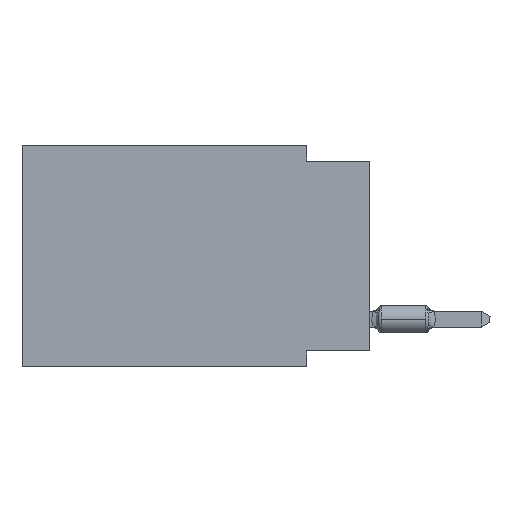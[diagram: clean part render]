
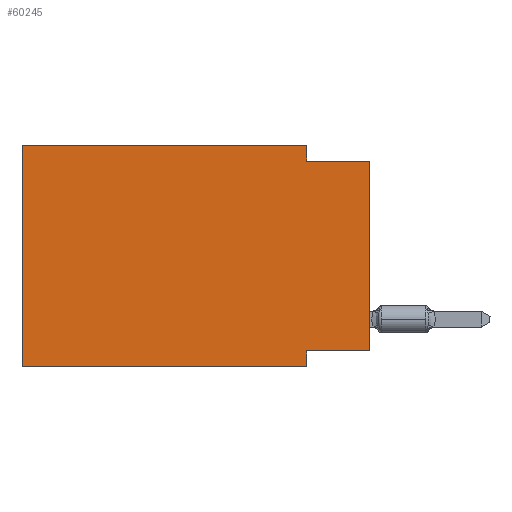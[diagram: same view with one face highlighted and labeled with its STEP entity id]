
A CAD part, left-side view. The second image highlights one B-rep face of the part: STEP entity #60245.
In plain terms, the highlighted planar face has unit normal (-1, 0, 0).
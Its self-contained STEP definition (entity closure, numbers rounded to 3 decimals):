
#179 = EDGE_CURVE ( 'NONE', #22009, #8965, #75726, .T. ) ;
#732 = VERTEX_POINT ( 'NONE', #2594 ) ;
#1118 = EDGE_CURVE ( 'NONE', #22180, #53012, #21975, .T. ) ;
#1610 = DIRECTION ( 'NONE',  ( 0., 0., 1. ) ) ;
#2594 = CARTESIAN_POINT ( 'NONE',  ( 0., 2.54, -8.255 ) ) ;
#3311 = CARTESIAN_POINT ( 'NONE',  ( 0., 13.97, -8.89 ) ) ;
#3717 = ORIENTED_EDGE ( 'NONE', *, *, #179, .F. ) ;
#4667 = CARTESIAN_POINT ( 'NONE',  ( 0., 13.97, 0. ) ) ;
#6177 = CARTESIAN_POINT ( 'NONE',  ( 0., 0., 0. ) ) ;
#6990 = VECTOR ( 'NONE', #15329, 1000. ) ;
#8965 = VERTEX_POINT ( 'NONE', #53309 ) ;
#9182 = CARTESIAN_POINT ( 'NONE',  ( 0., 2.54, -8.89 ) ) ;
#9951 = CARTESIAN_POINT ( 'NONE',  ( 0., 2.54, 0. ) ) ;
#10182 = VECTOR ( 'NONE', #56803, 1000. ) ;
#10287 = EDGE_CURVE ( 'NONE', #53012, #22009, #56669, .T. ) ;
#11692 = CARTESIAN_POINT ( 'NONE',  ( 0., 13.97, -8.89 ) ) ;
#12405 = DIRECTION ( 'NONE',  ( 0., 0., 1. ) ) ;
#13027 = VERTEX_POINT ( 'NONE', #26581 ) ;
#13114 = ORIENTED_EDGE ( 'NONE', *, *, #73516, .T. ) ;
#15329 = DIRECTION ( 'NONE',  ( 0., 0., -1. ) ) ;
#17705 = ORIENTED_EDGE ( 'NONE', *, *, #42274, .F. ) ;
#18898 = VECTOR ( 'NONE', #34586, 1000. ) ;
#19705 = DIRECTION ( 'NONE',  ( 0., 0., -1. ) ) ;
#19970 = CARTESIAN_POINT ( 'NONE',  ( 0., 0., -8.255 ) ) ;
#21975 = LINE ( 'NONE', #82127, #45866 ) ;
#22009 = VERTEX_POINT ( 'NONE', #9951 ) ;
#22180 = VERTEX_POINT ( 'NONE', #11692 ) ;
#22438 = ORIENTED_EDGE ( 'NONE', *, *, #78961, .T. ) ;
#23247 = DIRECTION ( 'NONE',  ( 0., -1., 0. ) ) ;
#24933 = CARTESIAN_POINT ( 'NONE',  ( 0., 0., -0.635 ) ) ;
#26581 = CARTESIAN_POINT ( 'NONE',  ( 0., 0., -0.635 ) ) ;
#28441 = VERTEX_POINT ( 'NONE', #19970 ) ;
#34586 = DIRECTION ( 'NONE',  ( 0., 0., -1. ) ) ;
#36046 = CARTESIAN_POINT ( 'NONE',  ( 0., 0., -8.255 ) ) ;
#37106 = CARTESIAN_POINT ( 'NONE',  ( 0., 13.97, 0. ) ) ;
#39161 = VECTOR ( 'NONE', #23247, 1000. ) ;
#39787 = AXIS2_PLACEMENT_3D ( 'NONE', #4667, #80297, #19705 ) ;
#41348 = ORIENTED_EDGE ( 'NONE', *, *, #79651, .F. ) ;
#41358 = LINE ( 'NONE', #36046, #68767 ) ;
#41888 = LINE ( 'NONE', #57322, #6990 ) ;
#42274 = EDGE_CURVE ( 'NONE', #732, #75362, #41888, .T. ) ;
#43846 = EDGE_LOOP ( 'NONE', ( #22438, #41348, #3717, #51243, #74874, #13114, #17705, #62508 ) ) ;
#45866 = VECTOR ( 'NONE', #1610, 1000. ) ;
#51101 = VECTOR ( 'NONE', #12405, 1000. ) ;
#51243 = ORIENTED_EDGE ( 'NONE', *, *, #10287, .F. ) ;
#52436 = PLANE ( 'NONE',  #39787 ) ;
#53012 = VERTEX_POINT ( 'NONE', #37106 ) ;
#53309 = CARTESIAN_POINT ( 'NONE',  ( 0., 2.54, -0.635 ) ) ;
#53840 = VECTOR ( 'NONE', #76574, 1000. ) ;
#56669 = LINE ( 'NONE', #77447, #53840 ) ;
#56803 = DIRECTION ( 'NONE',  ( 0., -1., 0. ) ) ;
#57322 = CARTESIAN_POINT ( 'NONE',  ( 0., 2.54, -8.89 ) ) ;
#58434 = LINE ( 'NONE', #6177, #51101 ) ;
#60245 = ADVANCED_FACE ( 'NONE', ( #65285 ), #52436, .F. ) ;
#62508 = ORIENTED_EDGE ( 'NONE', *, *, #85739, .F. ) ;
#65285 = FACE_OUTER_BOUND ( 'NONE', #43846, .T. ) ;
#68767 = VECTOR ( 'NONE', #75418, 1000. ) ;
#69092 = CARTESIAN_POINT ( 'NONE',  ( 0., 2.54, 0. ) ) ;
#73516 = EDGE_CURVE ( 'NONE', #22180, #75362, #83838, .T. ) ;
#74874 = ORIENTED_EDGE ( 'NONE', *, *, #1118, .F. ) ;
#75362 = VERTEX_POINT ( 'NONE', #9182 ) ;
#75418 = DIRECTION ( 'NONE',  ( 0., 1., 0. ) ) ;
#75726 = LINE ( 'NONE', #69092, #18898 ) ;
#76574 = DIRECTION ( 'NONE',  ( 0., -1., 0. ) ) ;
#77447 = CARTESIAN_POINT ( 'NONE',  ( 0., 13.97, 0. ) ) ;
#78961 = EDGE_CURVE ( 'NONE', #28441, #13027, #58434, .T. ) ;
#79651 = EDGE_CURVE ( 'NONE', #8965, #13027, #85525, .T. ) ;
#80297 = DIRECTION ( 'NONE',  ( 1., 0., 0. ) ) ;
#82127 = CARTESIAN_POINT ( 'NONE',  ( 0., 13.97, 0. ) ) ;
#83838 = LINE ( 'NONE', #3311, #39161 ) ;
#85525 = LINE ( 'NONE', #24933, #10182 ) ;
#85739 = EDGE_CURVE ( 'NONE', #28441, #732, #41358, .T. ) ;
